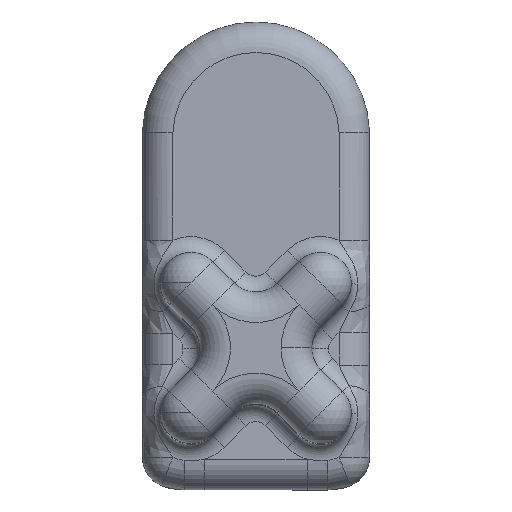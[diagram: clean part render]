
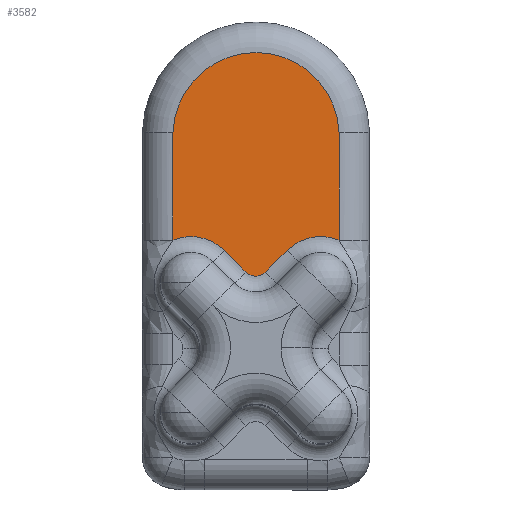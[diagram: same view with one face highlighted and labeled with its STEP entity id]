
A CAD part, top view. The second image highlights one B-rep face of the part: STEP entity #3582.
In plain terms, the highlighted planar face has unit normal (0, 0, 1).
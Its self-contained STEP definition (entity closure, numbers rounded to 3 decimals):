
#85 = DIRECTION ( 'NONE',  ( 0., 1., 0. ) ) ;
#156 = VECTOR ( 'NONE', #2989, 1000. ) ;
#200 = EDGE_CURVE ( 'NONE', #3151, #1840, #4333, .T. ) ;
#246 = EDGE_CURVE ( 'NONE', #1840, #651, #5342, .T. ) ;
#301 = EDGE_CURVE ( 'NONE', #651, #2947, #1483, .T. ) ;
#343 = EDGE_CURVE ( 'NONE', #2947, #2046, #1300, .T. ) ;
#379 = EDGE_CURVE ( 'NONE', #2046, #5985, #6161, .T. ) ;
#382 = AXIS2_PLACEMENT_3D ( 'NONE', #2581, #4102, #1004 ) ;
#389 = EDGE_CURVE ( 'NONE', #5985, #1652, #5066, .T. ) ;
#426 = EDGE_CURVE ( 'NONE', #1652, #3780, #4043, .T. ) ;
#440 = CARTESIAN_POINT ( 'NONE',  ( -8.618, 39.361, -22.818 ) ) ;
#520 = EDGE_CURVE ( 'NONE', #3780, #3151, #6032, .T. ) ;
#651 = VERTEX_POINT ( 'NONE', #1909 ) ;
#722 = ORIENTED_EDGE ( 'NONE', *, *, #343, .T. ) ;
#1004 = DIRECTION ( 'NONE',  ( 0., -1., 0. ) ) ;
#1054 = CARTESIAN_POINT ( 'NONE',  ( -8.618, 22.259, -22.818 ) ) ;
#1196 = ORIENTED_EDGE ( 'NONE', *, *, #389, .T. ) ;
#1300 = CIRCLE ( 'NONE', #5620, 7.75 ) ;
#1327 = ORIENTED_EDGE ( 'NONE', *, *, #520, .T. ) ;
#1483 = LINE ( 'NONE', #3163, #156 ) ;
#1652 = VERTEX_POINT ( 'NONE', #5920 ) ;
#1654 = VECTOR ( 'NONE', #85, 1000. ) ;
#1840 = VERTEX_POINT ( 'NONE', #5137 ) ;
#1909 = CARTESIAN_POINT ( 'NONE',  ( -35.751, 39.838, -22.818 ) ) ;
#2046 = VERTEX_POINT ( 'NONE', #4619 ) ;
#2078 = AXIS2_PLACEMENT_3D ( 'NONE', #2349, #2343, #2340 ) ;
#2098 = ORIENTED_EDGE ( 'NONE', *, *, #200, .T. ) ;
#2123 = CARTESIAN_POINT ( 'NONE',  ( -35.751, 22.29, -22.818 ) ) ;
#2300 = AXIS2_PLACEMENT_3D ( 'NONE', #2772, #2760, #2756 ) ;
#2340 = DIRECTION ( 'NONE',  ( 1., 0., 0. ) ) ;
#2343 = DIRECTION ( 'NONE',  ( 0., 0., -1. ) ) ;
#2349 = CARTESIAN_POINT ( 'NONE',  ( -11.616, 15.112, -22.818 ) ) ;
#2508 = EDGE_LOOP ( 'NONE', ( #1327, #2098, #6105, #3786, #722, #4359, #1196, #2936 ) ) ;
#2581 = CARTESIAN_POINT ( 'NONE',  ( -22.184, 39.361, -22.818 ) ) ;
#2583 = DIRECTION ( 'NONE',  ( 0.707, -0.707, 0. ) ) ;
#2703 = DIRECTION ( 'NONE',  ( 0.707, 0.707, 0. ) ) ;
#2727 = CARTESIAN_POINT ( 'NONE',  ( -28.343, 9.345, -22.818 ) ) ;
#2756 = DIRECTION ( 'NONE',  ( 1., 0., 0. ) ) ;
#2760 = DIRECTION ( 'NONE',  ( 0., 0., 1. ) ) ;
#2772 = CARTESIAN_POINT ( 'NONE',  ( -22.222, 18.648, -22.818 ) ) ;
#2839 = CARTESIAN_POINT ( 'NONE',  ( -4.347, -2.41, -22.818 ) ) ;
#2846 = DIRECTION ( 'NONE',  ( 1., 0., 0. ) ) ;
#2852 = DIRECTION ( 'NONE',  ( 0., 0., -1. ) ) ;
#2862 = CARTESIAN_POINT ( 'NONE',  ( -32.829, 15.112, -22.818 ) ) ;
#2936 = ORIENTED_EDGE ( 'NONE', *, *, #426, .T. ) ;
#2947 = VERTEX_POINT ( 'NONE', #2123 ) ;
#2989 = DIRECTION ( 'NONE',  ( 0., -1., 0. ) ) ;
#3151 = VERTEX_POINT ( 'NONE', #1054 ) ;
#3163 = CARTESIAN_POINT ( 'NONE',  ( -35.751, 39.361, -22.818 ) ) ;
#3177 = DIRECTION ( 'NONE',  ( -1., 0., 0. ) ) ;
#3199 = DIRECTION ( 'NONE',  ( 0., 0., 1. ) ) ;
#3202 = CARTESIAN_POINT ( 'NONE',  ( -22.184, 39.361, -22.818 ) ) ;
#3582 = ADVANCED_FACE ( 'NONE', ( #5495 ), #3635, .F. ) ;
#3635 = PLANE ( 'NONE',  #382 ) ;
#3780 = VERTEX_POINT ( 'NONE', #4602 ) ;
#3786 = ORIENTED_EDGE ( 'NONE', *, *, #301, .T. ) ;
#3896 = VECTOR ( 'NONE', #2583, 1000. ) ;
#4043 = LINE ( 'NONE', #2727, #4936 ) ;
#4102 = DIRECTION ( 'NONE',  ( 0., 0., -1. ) ) ;
#4177 = CARTESIAN_POINT ( 'NONE',  ( -23.813, 17.057, -22.818 ) ) ;
#4333 = LINE ( 'NONE', #440, #1654 ) ;
#4359 = ORIENTED_EDGE ( 'NONE', *, *, #379, .T. ) ;
#4602 = CARTESIAN_POINT ( 'NONE',  ( -17.096, 20.592, -22.818 ) ) ;
#4619 = CARTESIAN_POINT ( 'NONE',  ( -27.349, 20.592, -22.818 ) ) ;
#4648 = AXIS2_PLACEMENT_3D ( 'NONE', #3202, #3199, #3177 ) ;
#4936 = VECTOR ( 'NONE', #2703, 1000. ) ;
#5066 = CIRCLE ( 'NONE', #2300, 2.25 ) ;
#5137 = CARTESIAN_POINT ( 'NONE',  ( -8.618, 39.838, -22.818 ) ) ;
#5342 = CIRCLE ( 'NONE', #4648, 13.575 ) ;
#5495 = FACE_OUTER_BOUND ( 'NONE', #2508, .T. ) ;
#5620 = AXIS2_PLACEMENT_3D ( 'NONE', #2862, #2852, #2846 ) ;
#5920 = CARTESIAN_POINT ( 'NONE',  ( -20.631, 17.057, -22.818 ) ) ;
#5985 = VERTEX_POINT ( 'NONE', #4177 ) ;
#6032 = CIRCLE ( 'NONE', #2078, 7.75 ) ;
#6105 = ORIENTED_EDGE ( 'NONE', *, *, #246, .T. ) ;
#6161 = LINE ( 'NONE', #2839, #3896 ) ;
